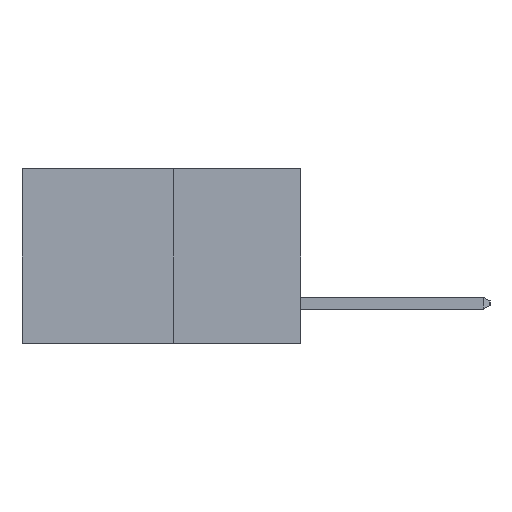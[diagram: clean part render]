
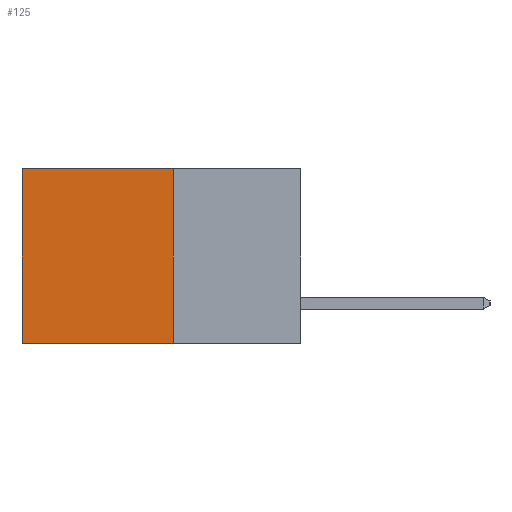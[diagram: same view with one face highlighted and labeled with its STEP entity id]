
A CAD part, left-side view. The second image highlights one B-rep face of the part: STEP entity #125.
In plain terms, the highlighted planar face has unit normal (-1, 0, 0).
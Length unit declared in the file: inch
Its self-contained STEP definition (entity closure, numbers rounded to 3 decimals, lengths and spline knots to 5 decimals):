
#125 = ADVANCED_FACE ( 'NONE', ( #2408 ), #17229, .F. ) ;
#518 = VERTEX_POINT ( 'NONE', #5891 ) ;
#584 = DIRECTION ( 'NONE',  ( 0., 1., 0. ) ) ;
#753 = EDGE_CURVE ( 'NONE', #10517, #1207, #16539, .T. ) ;
#1207 = VERTEX_POINT ( 'NONE', #14491 ) ;
#2406 = CARTESIAN_POINT ( 'NONE',  ( 0.277, 0.59, 0. ) ) ;
#2408 = FACE_OUTER_BOUND ( 'NONE', #4815, .T. ) ;
#4192 = VECTOR ( 'NONE', #584, 39.37008 ) ;
#4712 = LINE ( 'NONE', #7336, #4192 ) ;
#4815 = EDGE_LOOP ( 'NONE', ( #20222, #7949, #17880, #18254 ) ) ;
#5891 = CARTESIAN_POINT ( 'NONE',  ( 0.277, 0.27, 0. ) ) ;
#6037 = CARTESIAN_POINT ( 'NONE',  ( 0.277, 0.27, -0.37 ) ) ;
#6504 = VECTOR ( 'NONE', #13468, 39.37008 ) ;
#7336 = CARTESIAN_POINT ( 'NONE',  ( 0.277, 0.27, 0. ) ) ;
#7542 = DIRECTION ( 'NONE',  ( 0., 0., -1. ) ) ;
#7949 = ORIENTED_EDGE ( 'NONE', *, *, #14628, .F. ) ;
#8722 = AXIS2_PLACEMENT_3D ( 'NONE', #18684, #16554, #7542 ) ;
#9635 = VERTEX_POINT ( 'NONE', #6037 ) ;
#9719 = DIRECTION ( 'NONE',  ( 0., 1., 0. ) ) ;
#10104 = CARTESIAN_POINT ( 'NONE',  ( 0.277, 0.27, -0.37 ) ) ;
#10517 = VERTEX_POINT ( 'NONE', #2406 ) ;
#10923 = LINE ( 'NONE', #10104, #6504 ) ;
#12902 = CARTESIAN_POINT ( 'NONE',  ( 0.277, 0.59, -0.37 ) ) ;
#13391 = DIRECTION ( 'NONE',  ( 0., 0., -1. ) ) ;
#13468 = DIRECTION ( 'NONE',  ( 0., 0., -1. ) ) ;
#14332 = EDGE_CURVE ( 'NONE', #518, #10517, #4712, .T. ) ;
#14491 = CARTESIAN_POINT ( 'NONE',  ( 0.277, 0.59, -0.37 ) ) ;
#14628 = EDGE_CURVE ( 'NONE', #9635, #1207, #20134, .T. ) ;
#16026 = VECTOR ( 'NONE', #13391, 39.37008 ) ;
#16539 = LINE ( 'NONE', #12902, #16026 ) ;
#16554 = DIRECTION ( 'NONE',  ( 1., 0., 0. ) ) ;
#17229 = PLANE ( 'NONE',  #8722 ) ;
#17880 = ORIENTED_EDGE ( 'NONE', *, *, #21346, .F. ) ;
#18254 = ORIENTED_EDGE ( 'NONE', *, *, #14332, .T. ) ;
#18684 = CARTESIAN_POINT ( 'NONE',  ( 0.277, 0.27, -0.37 ) ) ;
#20134 = LINE ( 'NONE', #21419, #20655 ) ;
#20222 = ORIENTED_EDGE ( 'NONE', *, *, #753, .T. ) ;
#20655 = VECTOR ( 'NONE', #9719, 39.37008 ) ;
#21346 = EDGE_CURVE ( 'NONE', #518, #9635, #10923, .T. ) ;
#21419 = CARTESIAN_POINT ( 'NONE',  ( 0.277, 0.27, -0.37 ) ) ;
